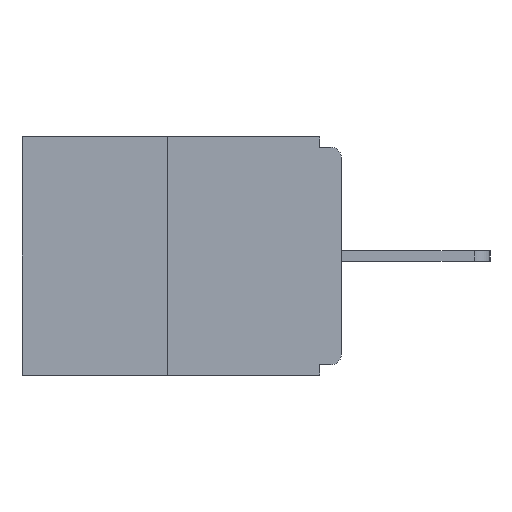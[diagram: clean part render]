
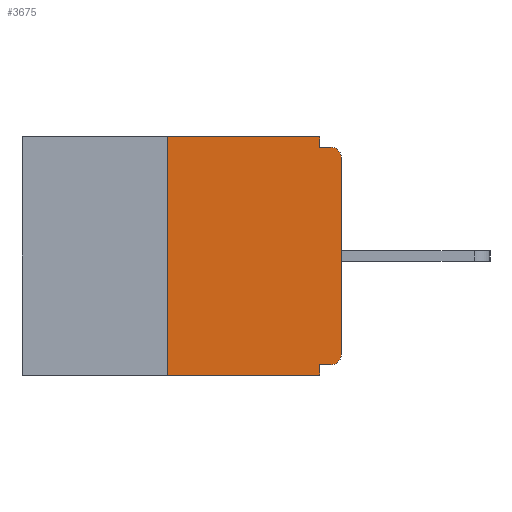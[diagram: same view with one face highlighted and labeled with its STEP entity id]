
A CAD part, left-side view. The second image highlights one B-rep face of the part: STEP entity #3675.
In plain terms, the highlighted planar face has unit normal (-1, 0, 0).
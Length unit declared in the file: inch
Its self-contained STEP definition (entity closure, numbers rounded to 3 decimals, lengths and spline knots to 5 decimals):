
#165 = EDGE_CURVE ( 'NONE', #10232, #5994, #14020, .T. ) ;
#169 = ORIENTED_EDGE ( 'NONE', *, *, #3482, .F. ) ;
#516 = CARTESIAN_POINT ( 'NONE',  ( 0., 0., -0.313 ) ) ;
#527 = CARTESIAN_POINT ( 'NONE',  ( 0., 0.46, -0.343 ) ) ;
#1482 = VECTOR ( 'NONE', #11276, 39.37008 ) ;
#1652 = CARTESIAN_POINT ( 'NONE',  ( 0., 0.46, 0. ) ) ;
#1929 = EDGE_CURVE ( 'NONE', #6217, #15129, #8779, .T. ) ;
#2119 = CIRCLE ( 'NONE', #3199, 0.015 ) ;
#2224 = DIRECTION ( 'NONE',  ( 0., 1., 0. ) ) ;
#2235 = LINE ( 'NONE', #17784, #9887 ) ;
#2545 = VECTOR ( 'NONE', #13809, 39.37008 ) ;
#2988 = CARTESIAN_POINT ( 'NONE',  ( 0., 0.25, 0. ) ) ;
#3029 = CARTESIAN_POINT ( 'NONE',  ( 0., 0.015, -0.328 ) ) ;
#3153 = CARTESIAN_POINT ( 'NONE',  ( 0., 0.031, -0.343 ) ) ;
#3199 = AXIS2_PLACEMENT_3D ( 'NONE', #5201, #15703, #6760 ) ;
#3482 = EDGE_CURVE ( 'NONE', #14753, #5244, #16815, .T. ) ;
#3675 = ADVANCED_FACE ( 'NONE', ( #6099 ), #3978, .F. ) ;
#3865 = LINE ( 'NONE', #11358, #19193 ) ;
#3906 = DIRECTION ( 'NONE',  ( 1., 0., 0. ) ) ;
#3978 = PLANE ( 'NONE',  #7597 ) ;
#4554 = DIRECTION ( 'NONE',  ( 0., 0., -1. ) ) ;
#4919 = VECTOR ( 'NONE', #18959, 39.37008 ) ;
#5201 = CARTESIAN_POINT ( 'NONE',  ( 0., 0.015, -0.313 ) ) ;
#5244 = VERTEX_POINT ( 'NONE', #2988 ) ;
#5245 = VERTEX_POINT ( 'NONE', #3029 ) ;
#5979 = VERTEX_POINT ( 'NONE', #8187 ) ;
#5994 = VERTEX_POINT ( 'NONE', #17102 ) ;
#6099 = FACE_OUTER_BOUND ( 'NONE', #9485, .T. ) ;
#6217 = VERTEX_POINT ( 'NONE', #516 ) ;
#6246 = DIRECTION ( 'NONE',  ( 0., 0., -1. ) ) ;
#6354 = CARTESIAN_POINT ( 'NONE',  ( 0., 0.015, -0.03 ) ) ;
#6527 = CARTESIAN_POINT ( 'NONE',  ( 0., 0.25, -0.343 ) ) ;
#6760 = DIRECTION ( 'NONE',  ( 0., 0., -1. ) ) ;
#6992 = EDGE_CURVE ( 'NONE', #16792, #10232, #2235, .T. ) ;
#7009 = ORIENTED_EDGE ( 'NONE', *, *, #10908, .F. ) ;
#7095 = EDGE_CURVE ( 'NONE', #13738, #5979, #15475, .T. ) ;
#7597 = AXIS2_PLACEMENT_3D ( 'NONE', #9365, #3906, #4554 ) ;
#7718 = DIRECTION ( 'NONE',  ( 0., 0., 1. ) ) ;
#7877 = DIRECTION ( 'NONE',  ( 0., 0., -1. ) ) ;
#7980 = CARTESIAN_POINT ( 'NONE',  ( 0., 0., -0.015 ) ) ;
#8187 = CARTESIAN_POINT ( 'NONE',  ( 0., 0.031, -0.343 ) ) ;
#8658 = ORIENTED_EDGE ( 'NONE', *, *, #9594, .T. ) ;
#8779 = LINE ( 'NONE', #12701, #16658 ) ;
#9365 = CARTESIAN_POINT ( 'NONE',  ( 0., 0.46, 0. ) ) ;
#9485 = EDGE_LOOP ( 'NONE', ( #7009, #169, #10290, #14736, #18991, #8658, #16981, #17884, #10997, #12410 ) ) ;
#9594 = EDGE_CURVE ( 'NONE', #5245, #6217, #2119, .T. ) ;
#9713 = LINE ( 'NONE', #1652, #2545 ) ;
#9887 = VECTOR ( 'NONE', #14899, 39.37008 ) ;
#10049 = VECTOR ( 'NONE', #18635, 39.37008 ) ;
#10232 = VERTEX_POINT ( 'NONE', #10694 ) ;
#10290 = ORIENTED_EDGE ( 'NONE', *, *, #18680, .T. ) ;
#10694 = CARTESIAN_POINT ( 'NONE',  ( 0., 0.031, -0.015 ) ) ;
#10908 = EDGE_CURVE ( 'NONE', #5244, #16792, #9713, .T. ) ;
#10997 = ORIENTED_EDGE ( 'NONE', *, *, #165, .F. ) ;
#11276 = DIRECTION ( 'NONE',  ( 0., -1., 0. ) ) ;
#11358 = CARTESIAN_POINT ( 'NONE',  ( 0., 0., -0.328 ) ) ;
#11544 = VECTOR ( 'NONE', #6246, 39.37008 ) ;
#11668 = CARTESIAN_POINT ( 'NONE',  ( 0., 0.031, 0. ) ) ;
#12410 = ORIENTED_EDGE ( 'NONE', *, *, #6992, .F. ) ;
#12701 = CARTESIAN_POINT ( 'NONE',  ( 0., 0., 0. ) ) ;
#12989 = AXIS2_PLACEMENT_3D ( 'NONE', #6354, #16758, #7877 ) ;
#13738 = VERTEX_POINT ( 'NONE', #18937 ) ;
#13809 = DIRECTION ( 'NONE',  ( 0., -1., 0. ) ) ;
#14020 = LINE ( 'NONE', #7980, #10049 ) ;
#14114 = LINE ( 'NONE', #527, #1482 ) ;
#14736 = ORIENTED_EDGE ( 'NONE', *, *, #7095, .F. ) ;
#14753 = VERTEX_POINT ( 'NONE', #6527 ) ;
#14899 = DIRECTION ( 'NONE',  ( 0., 0., -1. ) ) ;
#15129 = VERTEX_POINT ( 'NONE', #17705 ) ;
#15328 = EDGE_CURVE ( 'NONE', #15129, #5994, #16727, .T. ) ;
#15475 = LINE ( 'NONE', #3153, #11544 ) ;
#15703 = DIRECTION ( 'NONE',  ( -1., 0., 0. ) ) ;
#16090 = EDGE_CURVE ( 'NONE', #5245, #13738, #3865, .T. ) ;
#16658 = VECTOR ( 'NONE', #7718, 39.37008 ) ;
#16727 = CIRCLE ( 'NONE', #12989, 0.015 ) ;
#16758 = DIRECTION ( 'NONE',  ( -1., 0., 0. ) ) ;
#16792 = VERTEX_POINT ( 'NONE', #11668 ) ;
#16815 = LINE ( 'NONE', #19205, #4919 ) ;
#16981 = ORIENTED_EDGE ( 'NONE', *, *, #1929, .T. ) ;
#17102 = CARTESIAN_POINT ( 'NONE',  ( 0., 0.015, -0.015 ) ) ;
#17705 = CARTESIAN_POINT ( 'NONE',  ( 0., 0., -0.03 ) ) ;
#17784 = CARTESIAN_POINT ( 'NONE',  ( 0., 0.031, 0. ) ) ;
#17884 = ORIENTED_EDGE ( 'NONE', *, *, #15328, .T. ) ;
#18635 = DIRECTION ( 'NONE',  ( 0., -1., 0. ) ) ;
#18680 = EDGE_CURVE ( 'NONE', #14753, #5979, #14114, .T. ) ;
#18937 = CARTESIAN_POINT ( 'NONE',  ( 0., 0.031, -0.328 ) ) ;
#18959 = DIRECTION ( 'NONE',  ( 0., 0., 1. ) ) ;
#18991 = ORIENTED_EDGE ( 'NONE', *, *, #16090, .F. ) ;
#19193 = VECTOR ( 'NONE', #2224, 39.37008 ) ;
#19205 = CARTESIAN_POINT ( 'NONE',  ( 0., 0.25, 0. ) ) ;
